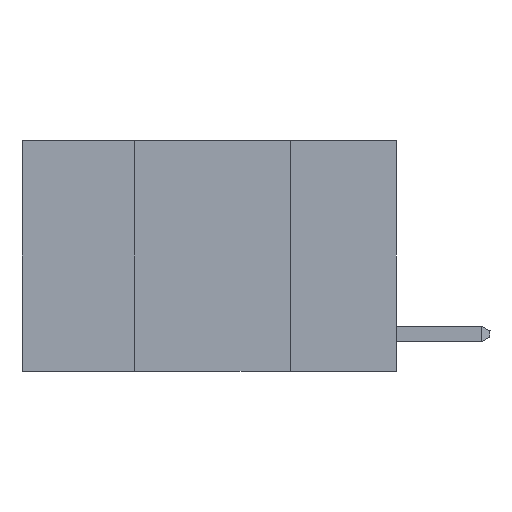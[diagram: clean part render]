
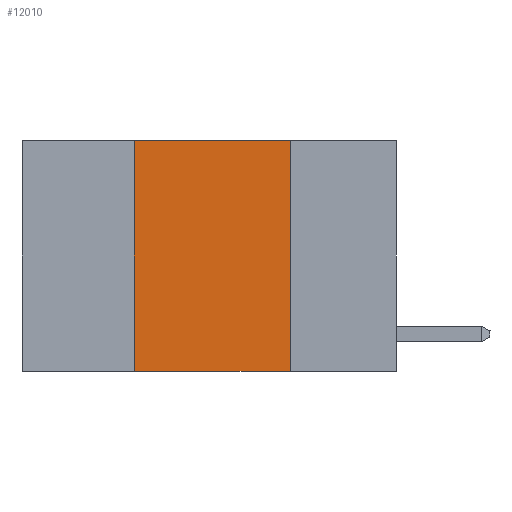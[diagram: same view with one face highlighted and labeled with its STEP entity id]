
A CAD part, left-side view. The second image highlights one B-rep face of the part: STEP entity #12010.
In plain terms, the highlighted planar face has unit normal (-1, 0, 0).
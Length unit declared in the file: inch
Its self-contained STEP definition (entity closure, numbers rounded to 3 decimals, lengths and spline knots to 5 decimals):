
#449 = LINE ( 'NONE', #5032, #5402 ) ;
#558 = DIRECTION ( 'NONE',  ( 1., 0., 0. ) ) ;
#1017 = EDGE_CURVE ( 'NONE', #5292, #6349, #5466, .T. ) ;
#1036 = EDGE_CURVE ( 'NONE', #11249, #9249, #10213, .T. ) ;
#1162 = VECTOR ( 'NONE', #2701, 39.37008 ) ;
#1254 = FACE_OUTER_BOUND ( 'NONE', #4421, .T. ) ;
#1316 = CARTESIAN_POINT ( 'NONE',  ( 0., 0.17, -0.37 ) ) ;
#1635 = ORIENTED_EDGE ( 'NONE', *, *, #7981, .F. ) ;
#2013 = LINE ( 'NONE', #2487, #9099 ) ;
#2487 = CARTESIAN_POINT ( 'NONE',  ( 0., 0.6, 0. ) ) ;
#2701 = DIRECTION ( 'NONE',  ( 0., 0., -1. ) ) ;
#3652 = EDGE_CURVE ( 'NONE', #11249, #6349, #449, .T. ) ;
#4421 = EDGE_LOOP ( 'NONE', ( #6002, #1635, #10573, #11404 ) ) ;
#4646 = CARTESIAN_POINT ( 'NONE',  ( 0., 0.17, 0. ) ) ;
#4743 = PLANE ( 'NONE',  #10692 ) ;
#5032 = CARTESIAN_POINT ( 'NONE',  ( 0., 0.6, -0.37 ) ) ;
#5262 = DIRECTION ( 'NONE',  ( 0., -1., 0. ) ) ;
#5292 = VERTEX_POINT ( 'NONE', #6655 ) ;
#5402 = VECTOR ( 'NONE', #5262, 39.37008 ) ;
#5466 = LINE ( 'NONE', #4646, #1162 ) ;
#6002 = ORIENTED_EDGE ( 'NONE', *, *, #1017, .F. ) ;
#6349 = VERTEX_POINT ( 'NONE', #1316 ) ;
#6655 = CARTESIAN_POINT ( 'NONE',  ( 0., 0.17, 0. ) ) ;
#6898 = CARTESIAN_POINT ( 'NONE',  ( 0., 0.6, 0. ) ) ;
#7981 = EDGE_CURVE ( 'NONE', #9249, #5292, #2013, .T. ) ;
#8928 = CARTESIAN_POINT ( 'NONE',  ( 0., 0.42, 0. ) ) ;
#9099 = VECTOR ( 'NONE', #13032, 39.37008 ) ;
#9249 = VERTEX_POINT ( 'NONE', #12034 ) ;
#9311 = DIRECTION ( 'NONE',  ( 0., 0., -1. ) ) ;
#10213 = LINE ( 'NONE', #8928, #12794 ) ;
#10573 = ORIENTED_EDGE ( 'NONE', *, *, #1036, .F. ) ;
#10692 = AXIS2_PLACEMENT_3D ( 'NONE', #6898, #558, #9311 ) ;
#11249 = VERTEX_POINT ( 'NONE', #12986 ) ;
#11404 = ORIENTED_EDGE ( 'NONE', *, *, #3652, .T. ) ;
#11989 = DIRECTION ( 'NONE',  ( 0., 0., 1. ) ) ;
#12010 = ADVANCED_FACE ( 'NONE', ( #1254 ), #4743, .F. ) ;
#12034 = CARTESIAN_POINT ( 'NONE',  ( 0., 0.42, 0. ) ) ;
#12794 = VECTOR ( 'NONE', #11989, 39.37008 ) ;
#12986 = CARTESIAN_POINT ( 'NONE',  ( 0., 0.42, -0.37 ) ) ;
#13032 = DIRECTION ( 'NONE',  ( 0., -1., 0. ) ) ;
